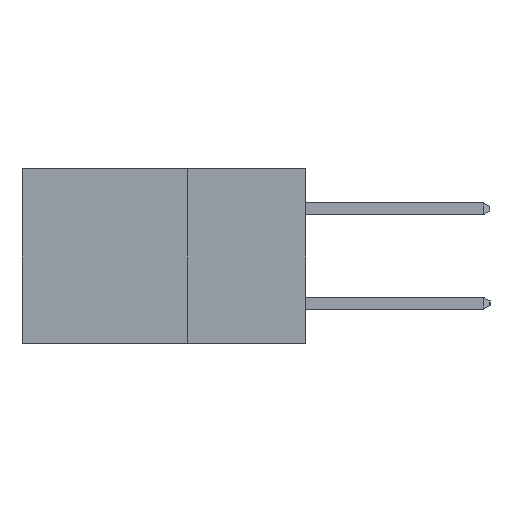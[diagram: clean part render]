
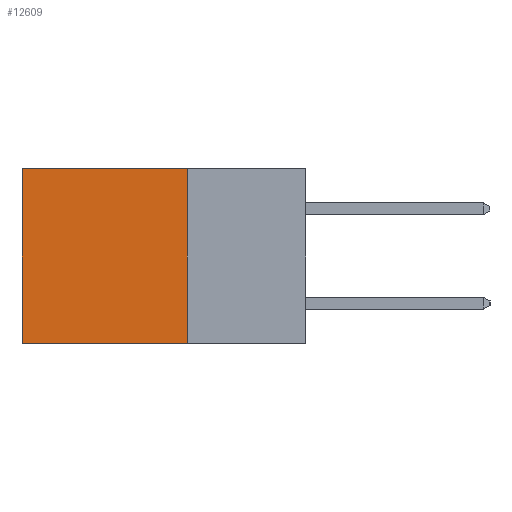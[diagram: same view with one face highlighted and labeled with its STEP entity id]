
A CAD part, left-side view. The second image highlights one B-rep face of the part: STEP entity #12609.
In plain terms, the highlighted planar face has unit normal (-1, 0, 0).
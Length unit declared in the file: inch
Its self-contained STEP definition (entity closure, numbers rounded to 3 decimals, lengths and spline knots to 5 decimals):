
#177 = CARTESIAN_POINT ( 'NONE',  ( 0.2615, 0.25, -0.37 ) ) ;
#235 = CARTESIAN_POINT ( 'NONE',  ( 0.2615, 0.25, 0. ) ) ;
#883 = VERTEX_POINT ( 'NONE', #235 ) ;
#1395 = VECTOR ( 'NONE', #9674, 39.37008 ) ;
#1556 = EDGE_CURVE ( 'NONE', #11041, #6384, #6070, .T. ) ;
#1954 = CARTESIAN_POINT ( 'NONE',  ( 0.2615, 0.25, -0.37 ) ) ;
#2331 = VECTOR ( 'NONE', #5023, 39.37008 ) ;
#2716 = DIRECTION ( 'NONE',  ( 0., 1., 0. ) ) ;
#3149 = DIRECTION ( 'NONE',  ( 1., 0., 0. ) ) ;
#3224 = ORIENTED_EDGE ( 'NONE', *, *, #11802, .F. ) ;
#3590 = ORIENTED_EDGE ( 'NONE', *, *, #7346, .F. ) ;
#4193 = LINE ( 'NONE', #9634, #10079 ) ;
#4451 = CARTESIAN_POINT ( 'NONE',  ( 0.2615, 0.25, 0. ) ) ;
#4473 = LINE ( 'NONE', #10069, #1395 ) ;
#4607 = AXIS2_PLACEMENT_3D ( 'NONE', #1954, #3149, #10877 ) ;
#4877 = LINE ( 'NONE', #4451, #10361 ) ;
#5023 = DIRECTION ( 'NONE',  ( 0., 0., -1. ) ) ;
#6053 = EDGE_CURVE ( 'NONE', #883, #11041, #4877, .T. ) ;
#6070 = LINE ( 'NONE', #10144, #2331 ) ;
#6339 = DIRECTION ( 'NONE',  ( 0., 1., 0. ) ) ;
#6349 = VERTEX_POINT ( 'NONE', #177 ) ;
#6384 = VERTEX_POINT ( 'NONE', #12479 ) ;
#7346 = EDGE_CURVE ( 'NONE', #883, #6349, #4473, .T. ) ;
#7676 = EDGE_LOOP ( 'NONE', ( #11322, #3224, #3590, #8307 ) ) ;
#8307 = ORIENTED_EDGE ( 'NONE', *, *, #6053, .T. ) ;
#8724 = PLANE ( 'NONE',  #4607 ) ;
#9403 = CARTESIAN_POINT ( 'NONE',  ( 0.2615, 0.6, 0. ) ) ;
#9634 = CARTESIAN_POINT ( 'NONE',  ( 0.2615, 0.25, -0.37 ) ) ;
#9674 = DIRECTION ( 'NONE',  ( 0., 0., -1. ) ) ;
#10069 = CARTESIAN_POINT ( 'NONE',  ( 0.2615, 0.25, -0.37 ) ) ;
#10079 = VECTOR ( 'NONE', #6339, 39.37008 ) ;
#10144 = CARTESIAN_POINT ( 'NONE',  ( 0.2615, 0.6, -0.37 ) ) ;
#10361 = VECTOR ( 'NONE', #2716, 39.37008 ) ;
#10877 = DIRECTION ( 'NONE',  ( 0., 0., -1. ) ) ;
#11041 = VERTEX_POINT ( 'NONE', #9403 ) ;
#11322 = ORIENTED_EDGE ( 'NONE', *, *, #1556, .T. ) ;
#11802 = EDGE_CURVE ( 'NONE', #6349, #6384, #4193, .T. ) ;
#12479 = CARTESIAN_POINT ( 'NONE',  ( 0.2615, 0.6, -0.37 ) ) ;
#12609 = ADVANCED_FACE ( 'NONE', ( #13480 ), #8724, .F. ) ;
#13480 = FACE_OUTER_BOUND ( 'NONE', #7676, .T. ) ;
